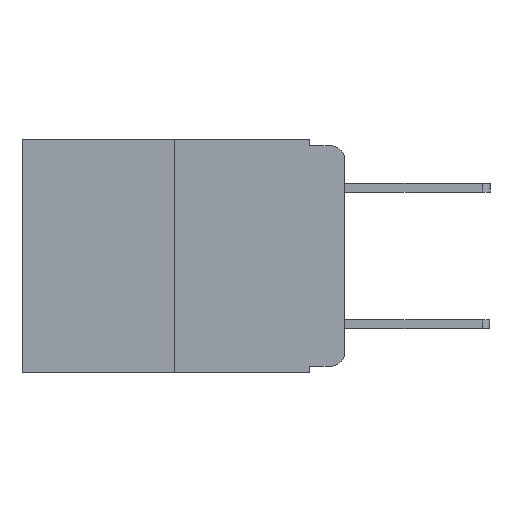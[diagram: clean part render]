
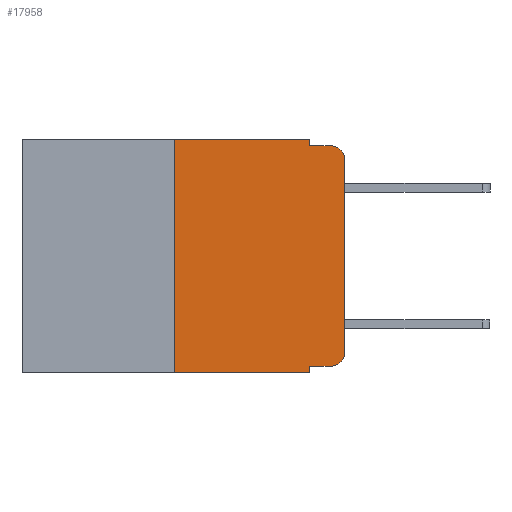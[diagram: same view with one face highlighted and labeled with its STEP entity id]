
A CAD part, left-side view. The second image highlights one B-rep face of the part: STEP entity #17958.
In plain terms, the highlighted planar face has unit normal (-1, 0, 0).
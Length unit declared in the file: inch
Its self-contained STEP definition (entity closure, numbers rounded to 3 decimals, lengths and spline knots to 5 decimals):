
#419 = ORIENTED_EDGE ( 'NONE', *, *, #1337, .T. ) ;
#756 = PLANE ( 'NONE',  #1466 ) ;
#1337 = EDGE_CURVE ( 'NONE', #12668, #7333, #2489, .T. ) ;
#1339 = CIRCLE ( 'NONE', #5279, 0.02 ) ;
#1353 = CARTESIAN_POINT ( 'NONE',  ( 0., 0.051, 0. ) ) ;
#1392 = LINE ( 'NONE', #23901, #6501 ) ;
#1466 = AXIS2_PLACEMENT_3D ( 'NONE', #12151, #2740, #15904 ) ;
#2014 = CARTESIAN_POINT ( 'NONE',  ( 0., 0.25, 0. ) ) ;
#2489 = CIRCLE ( 'NONE', #14562, 0.02 ) ;
#2704 = CARTESIAN_POINT ( 'NONE',  ( 0., 0.051, -0.343 ) ) ;
#2740 = DIRECTION ( 'NONE',  ( 1., 0., 0. ) ) ;
#2925 = CARTESIAN_POINT ( 'NONE',  ( 0., 0.051, -0.01 ) ) ;
#3007 = DIRECTION ( 'NONE',  ( 0., -1., 0. ) ) ;
#3040 = LINE ( 'NONE', #8396, #20616 ) ;
#3660 = ORIENTED_EDGE ( 'NONE', *, *, #5280, .F. ) ;
#3675 = CARTESIAN_POINT ( 'NONE',  ( 0., 0., 0. ) ) ;
#3843 = VERTEX_POINT ( 'NONE', #5873 ) ;
#4154 = EDGE_CURVE ( 'NONE', #8891, #7333, #14410, .T. ) ;
#4321 = EDGE_CURVE ( 'NONE', #7931, #13806, #1392, .T. ) ;
#4436 = EDGE_CURVE ( 'NONE', #21434, #12668, #23696, .T. ) ;
#4566 = ORIENTED_EDGE ( 'NONE', *, *, #4436, .T. ) ;
#5279 = AXIS2_PLACEMENT_3D ( 'NONE', #21480, #10351, #23329 ) ;
#5280 = EDGE_CURVE ( 'NONE', #16619, #18578, #24224, .T. ) ;
#5873 = CARTESIAN_POINT ( 'NONE',  ( 0., 0.25, -0.343 ) ) ;
#5912 = CARTESIAN_POINT ( 'NONE',  ( 0., 0., -0.03 ) ) ;
#6181 = VECTOR ( 'NONE', #23687, 39.37008 ) ;
#6501 = VECTOR ( 'NONE', #16565, 39.37008 ) ;
#6677 = ORIENTED_EDGE ( 'NONE', *, *, #13614, .T. ) ;
#6920 = CARTESIAN_POINT ( 'NONE',  ( 0., 0.473, -0.343 ) ) ;
#7333 = VERTEX_POINT ( 'NONE', #15733 ) ;
#7550 = CARTESIAN_POINT ( 'NONE',  ( 0., 0., -0.313 ) ) ;
#7604 = LINE ( 'NONE', #22575, #16346 ) ;
#7931 = VERTEX_POINT ( 'NONE', #2014 ) ;
#8313 = VECTOR ( 'NONE', #24211, 39.37008 ) ;
#8396 = CARTESIAN_POINT ( 'NONE',  ( 0., 0.051, 0. ) ) ;
#8891 = VERTEX_POINT ( 'NONE', #2925 ) ;
#9437 = VECTOR ( 'NONE', #3007, 39.37008 ) ;
#9675 = LINE ( 'NONE', #6920, #13487 ) ;
#9850 = CARTESIAN_POINT ( 'NONE',  ( 0., 0.051, 0. ) ) ;
#10351 = DIRECTION ( 'NONE',  ( -1., 0., 0. ) ) ;
#12034 = VERTEX_POINT ( 'NONE', #20848 ) ;
#12151 = CARTESIAN_POINT ( 'NONE',  ( 0., 0.473, 0. ) ) ;
#12668 = VERTEX_POINT ( 'NONE', #5912 ) ;
#12809 = ORIENTED_EDGE ( 'NONE', *, *, #16576, .T. ) ;
#13234 = DIRECTION ( 'NONE',  ( 0., 0., -1. ) ) ;
#13487 = VECTOR ( 'NONE', #18068, 39.37008 ) ;
#13614 = EDGE_CURVE ( 'NONE', #12034, #21434, #1339, .T. ) ;
#13684 = CARTESIAN_POINT ( 'NONE',  ( 0., 0.02, -0.03 ) ) ;
#13742 = EDGE_CURVE ( 'NONE', #3843, #18578, #9675, .T. ) ;
#13806 = VERTEX_POINT ( 'NONE', #1353 ) ;
#14077 = ORIENTED_EDGE ( 'NONE', *, *, #4154, .F. ) ;
#14288 = CARTESIAN_POINT ( 'NONE',  ( 0., 0.051, -0.01 ) ) ;
#14345 = EDGE_LOOP ( 'NONE', ( #4566, #419, #14077, #16138, #19332, #16728, #23443, #3660, #12809, #6677 ) ) ;
#14410 = LINE ( 'NONE', #14288, #9437 ) ;
#14562 = AXIS2_PLACEMENT_3D ( 'NONE', #13684, #19318, #13234 ) ;
#15095 = FACE_OUTER_BOUND ( 'NONE', #14345, .T. ) ;
#15294 = CARTESIAN_POINT ( 'NONE',  ( 0., 0.051, -0.333 ) ) ;
#15733 = CARTESIAN_POINT ( 'NONE',  ( 0., 0.02, -0.01 ) ) ;
#15827 = DIRECTION ( 'NONE',  ( 0., 0., -1. ) ) ;
#15904 = DIRECTION ( 'NONE',  ( 0., 0., -1. ) ) ;
#16138 = ORIENTED_EDGE ( 'NONE', *, *, #17944, .F. ) ;
#16346 = VECTOR ( 'NONE', #18862, 39.37008 ) ;
#16565 = DIRECTION ( 'NONE',  ( 0., -1., 0. ) ) ;
#16576 = EDGE_CURVE ( 'NONE', #16619, #12034, #7604, .T. ) ;
#16619 = VERTEX_POINT ( 'NONE', #15294 ) ;
#16728 = ORIENTED_EDGE ( 'NONE', *, *, #21214, .F. ) ;
#17359 = DIRECTION ( 'NONE',  ( 0., 0., -1. ) ) ;
#17944 = EDGE_CURVE ( 'NONE', #13806, #8891, #3040, .T. ) ;
#17958 = ADVANCED_FACE ( 'NONE', ( #15095 ), #756, .F. ) ;
#18068 = DIRECTION ( 'NONE',  ( 0., -1., 0. ) ) ;
#18578 = VERTEX_POINT ( 'NONE', #2704 ) ;
#18862 = DIRECTION ( 'NONE',  ( 0., -1., 0. ) ) ;
#19318 = DIRECTION ( 'NONE',  ( -1., 0., 0. ) ) ;
#19328 = VECTOR ( 'NONE', #17359, 39.37008 ) ;
#19332 = ORIENTED_EDGE ( 'NONE', *, *, #4321, .F. ) ;
#19979 = CARTESIAN_POINT ( 'NONE',  ( 0., 0.25, 0. ) ) ;
#20616 = VECTOR ( 'NONE', #15827, 39.37008 ) ;
#20848 = CARTESIAN_POINT ( 'NONE',  ( 0., 0.02, -0.333 ) ) ;
#21050 = LINE ( 'NONE', #19979, #6181 ) ;
#21214 = EDGE_CURVE ( 'NONE', #3843, #7931, #21050, .T. ) ;
#21434 = VERTEX_POINT ( 'NONE', #7550 ) ;
#21480 = CARTESIAN_POINT ( 'NONE',  ( 0., 0.02, -0.313 ) ) ;
#22575 = CARTESIAN_POINT ( 'NONE',  ( 0., 0.051, -0.333 ) ) ;
#23329 = DIRECTION ( 'NONE',  ( 0., 0., -1. ) ) ;
#23443 = ORIENTED_EDGE ( 'NONE', *, *, #13742, .T. ) ;
#23687 = DIRECTION ( 'NONE',  ( 0., 0., 1. ) ) ;
#23696 = LINE ( 'NONE', #3675, #8313 ) ;
#23901 = CARTESIAN_POINT ( 'NONE',  ( 0., 0.473, 0. ) ) ;
#24211 = DIRECTION ( 'NONE',  ( 0., 0., 1. ) ) ;
#24224 = LINE ( 'NONE', #9850, #19328 ) ;
